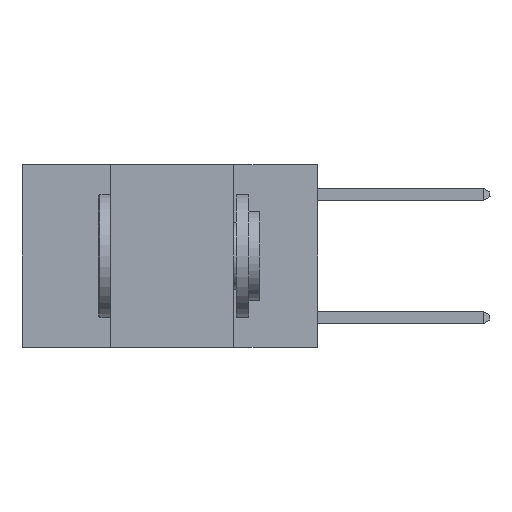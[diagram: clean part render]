
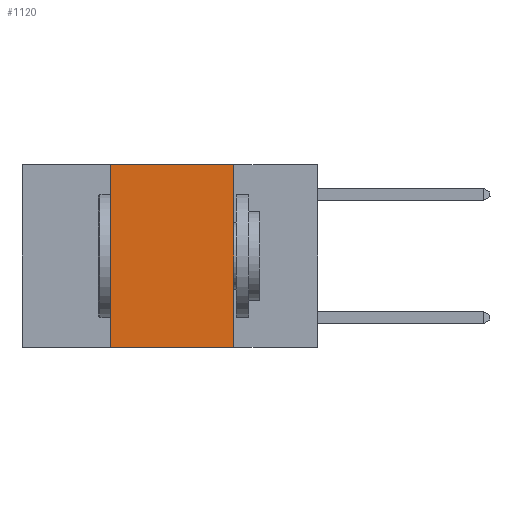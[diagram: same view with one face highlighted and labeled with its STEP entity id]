
A CAD part, left-side view. The second image highlights one B-rep face of the part: STEP entity #1120.
In plain terms, the highlighted planar face has unit normal (-1, 0, 0).
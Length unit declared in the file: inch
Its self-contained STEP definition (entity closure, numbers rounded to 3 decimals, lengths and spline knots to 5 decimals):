
#189 = EDGE_CURVE ( 'NONE', #2955, #11683, #28888, .T. ) ;
#868 = CARTESIAN_POINT ( 'NONE',  ( 0., 0.42, 0. ) ) ;
#1120 = ADVANCED_FACE ( 'NONE', ( #16645 ), #8320, .F. ) ;
#2001 = VERTEX_POINT ( 'NONE', #15667 ) ;
#2955 = VERTEX_POINT ( 'NONE', #26297 ) ;
#5753 = ORIENTED_EDGE ( 'NONE', *, *, #189, .F. ) ;
#5846 = VECTOR ( 'NONE', #23921, 39.37008 ) ;
#5907 = EDGE_LOOP ( 'NONE', ( #23388, #5753, #18700, #7932 ) ) ;
#6777 = VERTEX_POINT ( 'NONE', #21412 ) ;
#7932 = ORIENTED_EDGE ( 'NONE', *, *, #10950, .T. ) ;
#8098 = DIRECTION ( 'NONE',  ( 0., 0., -1. ) ) ;
#8200 = DIRECTION ( 'NONE',  ( 1., 0., 0. ) ) ;
#8290 = CARTESIAN_POINT ( 'NONE',  ( 0., 0.6, 0. ) ) ;
#8320 = PLANE ( 'NONE',  #17108 ) ;
#10557 = VECTOR ( 'NONE', #21951, 39.37008 ) ;
#10950 = EDGE_CURVE ( 'NONE', #6777, #2001, #23407, .T. ) ;
#10976 = LINE ( 'NONE', #18855, #27867 ) ;
#11683 = VERTEX_POINT ( 'NONE', #21796 ) ;
#13410 = LINE ( 'NONE', #868, #5846 ) ;
#15667 = CARTESIAN_POINT ( 'NONE',  ( 0., 0.17, -0.37 ) ) ;
#16645 = FACE_OUTER_BOUND ( 'NONE', #5907, .T. ) ;
#17108 = AXIS2_PLACEMENT_3D ( 'NONE', #8290, #8200, #8098 ) ;
#17117 = EDGE_CURVE ( 'NONE', #11683, #2001, #10976, .T. ) ;
#18649 = EDGE_CURVE ( 'NONE', #6777, #2955, #13410, .T. ) ;
#18700 = ORIENTED_EDGE ( 'NONE', *, *, #18649, .F. ) ;
#18855 = CARTESIAN_POINT ( 'NONE',  ( 0., 0.17, 0. ) ) ;
#21412 = CARTESIAN_POINT ( 'NONE',  ( 0., 0.42, -0.37 ) ) ;
#21631 = DIRECTION ( 'NONE',  ( 0., -1., 0. ) ) ;
#21796 = CARTESIAN_POINT ( 'NONE',  ( 0., 0.17, 0. ) ) ;
#21951 = DIRECTION ( 'NONE',  ( 0., -1., 0. ) ) ;
#22866 = CARTESIAN_POINT ( 'NONE',  ( 0., 0.6, 0. ) ) ;
#23388 = ORIENTED_EDGE ( 'NONE', *, *, #17117, .F. ) ;
#23407 = LINE ( 'NONE', #23950, #28780 ) ;
#23921 = DIRECTION ( 'NONE',  ( 0., 0., 1. ) ) ;
#23950 = CARTESIAN_POINT ( 'NONE',  ( 0., 0.6, -0.37 ) ) ;
#26297 = CARTESIAN_POINT ( 'NONE',  ( 0., 0.42, 0. ) ) ;
#27867 = VECTOR ( 'NONE', #28083, 39.37008 ) ;
#28083 = DIRECTION ( 'NONE',  ( 0., 0., -1. ) ) ;
#28780 = VECTOR ( 'NONE', #21631, 39.37008 ) ;
#28888 = LINE ( 'NONE', #22866, #10557 ) ;
